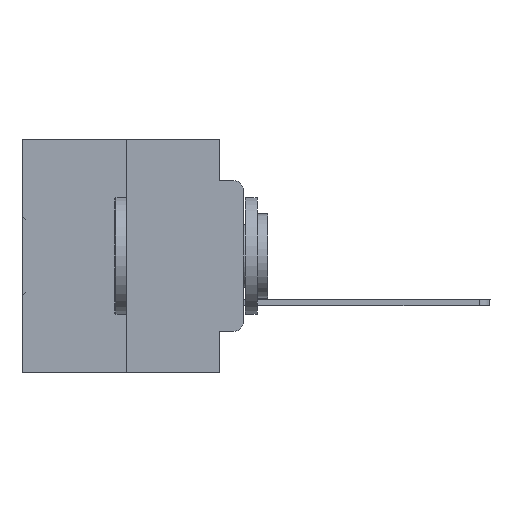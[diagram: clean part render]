
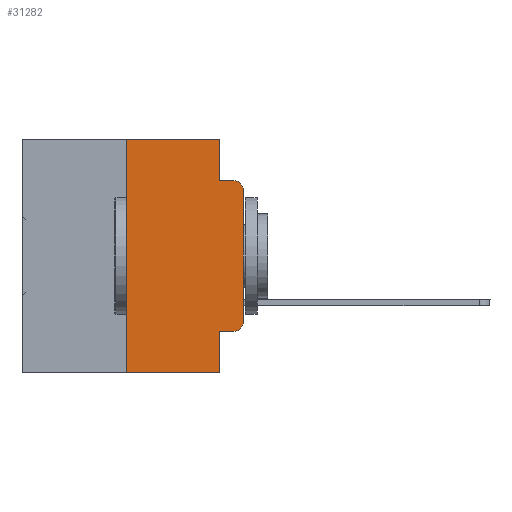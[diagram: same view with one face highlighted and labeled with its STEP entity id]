
A CAD part, left-side view. The second image highlights one B-rep face of the part: STEP entity #31282.
In plain terms, the highlighted planar face has unit normal (-1, 0, 0).
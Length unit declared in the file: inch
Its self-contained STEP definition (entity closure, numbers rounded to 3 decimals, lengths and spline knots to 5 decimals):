
#292 = AXIS2_PLACEMENT_3D ( 'NONE', #16170, #3362, #3868 ) ;
#1038 = CARTESIAN_POINT ( 'NONE',  ( 0., 0., -0.1085 ) ) ;
#1122 = CARTESIAN_POINT ( 'NONE',  ( 0., 0.25, -0.5 ) ) ;
#1852 = DIRECTION ( 'NONE',  ( 0., -1., 0. ) ) ;
#2115 = CARTESIAN_POINT ( 'NONE',  ( 0., 0.25, 0. ) ) ;
#2398 = ORIENTED_EDGE ( 'NONE', *, *, #5312, .T. ) ;
#2436 = ORIENTED_EDGE ( 'NONE', *, *, #4208, .F. ) ;
#2631 = ORIENTED_EDGE ( 'NONE', *, *, #29473, .F. ) ;
#3307 = CARTESIAN_POINT ( 'NONE',  ( 0., 0.02, -0.3915 ) ) ;
#3362 = DIRECTION ( 'NONE',  ( -1., 0., 0. ) ) ;
#3829 = LINE ( 'NONE', #14132, #28677 ) ;
#3868 = DIRECTION ( 'NONE',  ( 0., 0., -1. ) ) ;
#4208 = EDGE_CURVE ( 'NONE', #30108, #27108, #14612, .T. ) ;
#5210 = LINE ( 'NONE', #15491, #24290 ) ;
#5312 = EDGE_CURVE ( 'NONE', #16162, #27081, #24429, .T. ) ;
#5852 = VERTEX_POINT ( 'NONE', #24552 ) ;
#5997 = VERTEX_POINT ( 'NONE', #28552 ) ;
#6068 = DIRECTION ( 'NONE',  ( 1., 0., 0. ) ) ;
#6357 = ORIENTED_EDGE ( 'NONE', *, *, #26853, .T. ) ;
#6398 = ORIENTED_EDGE ( 'NONE', *, *, #30993, .F. ) ;
#6807 = EDGE_CURVE ( 'NONE', #30108, #5852, #24977, .T. ) ;
#7515 = CIRCLE ( 'NONE', #17207, 0.02 ) ;
#8354 = CIRCLE ( 'NONE', #292, 0.02 ) ;
#8575 = CARTESIAN_POINT ( 'NONE',  ( 0., 0.473, 0. ) ) ;
#9010 = EDGE_CURVE ( 'NONE', #27108, #27803, #5210, .T. ) ;
#9830 = LINE ( 'NONE', #30432, #23368 ) ;
#10102 = DIRECTION ( 'NONE',  ( 0., 0., -1. ) ) ;
#11095 = VERTEX_POINT ( 'NONE', #27796 ) ;
#11213 = EDGE_LOOP ( 'NONE', ( #2398, #22291, #6398, #18081, #26823, #2436, #25132, #2631, #6357, #23835 ) ) ;
#12413 = VERTEX_POINT ( 'NONE', #30354 ) ;
#13302 = DIRECTION ( 'NONE',  ( 0., -1., 0. ) ) ;
#13702 = CARTESIAN_POINT ( 'NONE',  ( 0., 0.25, 0. ) ) ;
#14132 = CARTESIAN_POINT ( 'NONE',  ( 0., 0.051, 0. ) ) ;
#14133 = CARTESIAN_POINT ( 'NONE',  ( 0., 0., 0. ) ) ;
#14558 = DIRECTION ( 'NONE',  ( 0., -1., 0. ) ) ;
#14612 = LINE ( 'NONE', #2115, #32296 ) ;
#15009 = CARTESIAN_POINT ( 'NONE',  ( 0., 0., -0.3915 ) ) ;
#15276 = EDGE_CURVE ( 'NONE', #27081, #12413, #8354, .T. ) ;
#15491 = CARTESIAN_POINT ( 'NONE',  ( 0., 0.473, 0. ) ) ;
#16162 = VERTEX_POINT ( 'NONE', #15009 ) ;
#16170 = CARTESIAN_POINT ( 'NONE',  ( 0., 0.02, -0.1085 ) ) ;
#16320 = DIRECTION ( 'NONE',  ( 0., 0., -1. ) ) ;
#16355 = CARTESIAN_POINT ( 'NONE',  ( 0., 0.051, -0.0885 ) ) ;
#16849 = LINE ( 'NONE', #16355, #29564 ) ;
#17207 = AXIS2_PLACEMENT_3D ( 'NONE', #3307, #26259, #26100 ) ;
#17369 = LINE ( 'NONE', #27839, #22192 ) ;
#18081 = ORIENTED_EDGE ( 'NONE', *, *, #18127, .F. ) ;
#18127 = EDGE_CURVE ( 'NONE', #27803, #5997, #3829, .T. ) ;
#19393 = CARTESIAN_POINT ( 'NONE',  ( 0., 0.473, -0.5 ) ) ;
#19873 = AXIS2_PLACEMENT_3D ( 'NONE', #8575, #6068, #29866 ) ;
#21250 = FACE_OUTER_BOUND ( 'NONE', #11213, .T. ) ;
#21293 = CARTESIAN_POINT ( 'NONE',  ( 0., 0.051, -0.4115 ) ) ;
#21837 = EDGE_CURVE ( 'NONE', #11095, #16162, #7515, .T. ) ;
#22192 = VECTOR ( 'NONE', #10102, 39.37008 ) ;
#22291 = ORIENTED_EDGE ( 'NONE', *, *, #15276, .T. ) ;
#23368 = VECTOR ( 'NONE', #14558, 39.37008 ) ;
#23835 = ORIENTED_EDGE ( 'NONE', *, *, #21837, .T. ) ;
#24290 = VECTOR ( 'NONE', #13302, 39.37008 ) ;
#24429 = LINE ( 'NONE', #14133, #25138 ) ;
#24552 = CARTESIAN_POINT ( 'NONE',  ( 0., 0.051, -0.5 ) ) ;
#24977 = LINE ( 'NONE', #19393, #28706 ) ;
#25077 = DIRECTION ( 'NONE',  ( 0., 0., 1. ) ) ;
#25132 = ORIENTED_EDGE ( 'NONE', *, *, #6807, .T. ) ;
#25138 = VECTOR ( 'NONE', #29164, 39.37008 ) ;
#26100 = DIRECTION ( 'NONE',  ( 0., 0., -1. ) ) ;
#26259 = DIRECTION ( 'NONE',  ( -1., 0., 0. ) ) ;
#26823 = ORIENTED_EDGE ( 'NONE', *, *, #9010, .F. ) ;
#26853 = EDGE_CURVE ( 'NONE', #27137, #11095, #9830, .T. ) ;
#27081 = VERTEX_POINT ( 'NONE', #1038 ) ;
#27108 = VERTEX_POINT ( 'NONE', #13702 ) ;
#27137 = VERTEX_POINT ( 'NONE', #21293 ) ;
#27796 = CARTESIAN_POINT ( 'NONE',  ( 0., 0.02, -0.4115 ) ) ;
#27803 = VERTEX_POINT ( 'NONE', #32785 ) ;
#27839 = CARTESIAN_POINT ( 'NONE',  ( 0., 0.051, 0. ) ) ;
#28552 = CARTESIAN_POINT ( 'NONE',  ( 0., 0.051, -0.0885 ) ) ;
#28677 = VECTOR ( 'NONE', #16320, 39.37008 ) ;
#28706 = VECTOR ( 'NONE', #1852, 39.37008 ) ;
#29164 = DIRECTION ( 'NONE',  ( 0., 0., 1. ) ) ;
#29473 = EDGE_CURVE ( 'NONE', #27137, #5852, #17369, .T. ) ;
#29564 = VECTOR ( 'NONE', #29699, 39.37008 ) ;
#29699 = DIRECTION ( 'NONE',  ( 0., -1., 0. ) ) ;
#29866 = DIRECTION ( 'NONE',  ( 0., 0., -1. ) ) ;
#30108 = VERTEX_POINT ( 'NONE', #1122 ) ;
#30354 = CARTESIAN_POINT ( 'NONE',  ( 0., 0.02, -0.0885 ) ) ;
#30432 = CARTESIAN_POINT ( 'NONE',  ( 0., 0.051, -0.4115 ) ) ;
#30993 = EDGE_CURVE ( 'NONE', #5997, #12413, #16849, .T. ) ;
#31282 = ADVANCED_FACE ( 'NONE', ( #21250 ), #31721, .F. ) ;
#31721 = PLANE ( 'NONE',  #19873 ) ;
#32296 = VECTOR ( 'NONE', #25077, 39.37008 ) ;
#32785 = CARTESIAN_POINT ( 'NONE',  ( 0., 0.051, 0. ) ) ;
